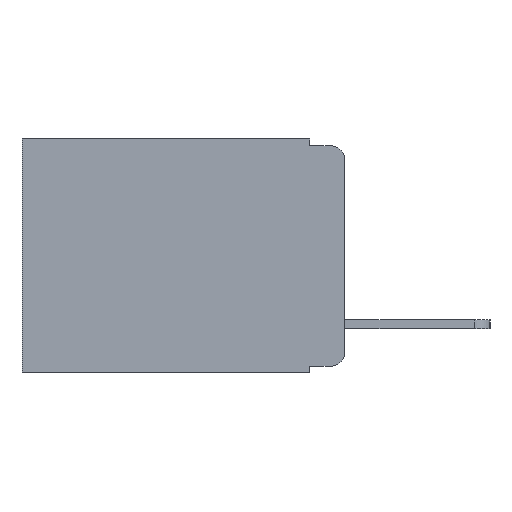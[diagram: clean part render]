
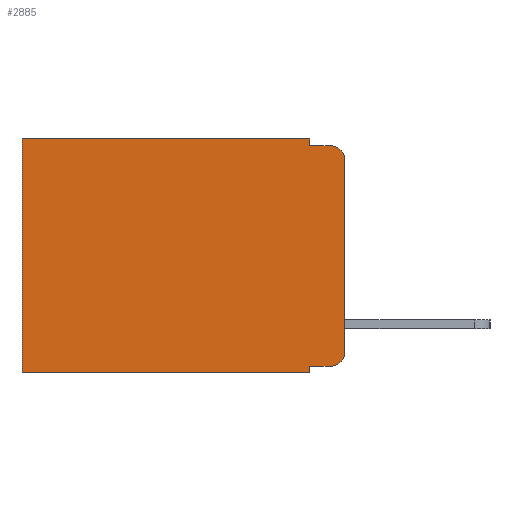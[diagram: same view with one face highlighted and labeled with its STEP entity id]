
A CAD part, left-side view. The second image highlights one B-rep face of the part: STEP entity #2885.
In plain terms, the highlighted planar face has unit normal (-1, 0, 0).
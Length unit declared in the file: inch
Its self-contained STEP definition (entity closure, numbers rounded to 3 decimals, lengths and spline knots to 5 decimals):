
#58 = ORIENTED_EDGE ( 'NONE', *, *, #12656, .T. ) ;
#78 = VECTOR ( 'NONE', #8382, 39.37008 ) ;
#124 = EDGE_CURVE ( 'NONE', #10309, #8480, #2674, .T. ) ;
#230 = CARTESIAN_POINT ( 'NONE',  ( 0.298, 0., 0. ) ) ;
#416 = CARTESIAN_POINT ( 'NONE',  ( 0.298, 0., -0.343 ) ) ;
#528 = DIRECTION ( 'NONE',  ( 0., 1., 0. ) ) ;
#673 = VERTEX_POINT ( 'NONE', #12947 ) ;
#687 = CARTESIAN_POINT ( 'NONE',  ( 0.298, 0., -0.03 ) ) ;
#918 = CARTESIAN_POINT ( 'NONE',  ( 0.298, 0.051, 0. ) ) ;
#926 = CARTESIAN_POINT ( 'NONE',  ( 0.298, 0.051, 0. ) ) ;
#1571 = CARTESIAN_POINT ( 'NONE',  ( 0.298, 0.473, 0. ) ) ;
#2151 = LINE ( 'NONE', #5682, #7761 ) ;
#2384 = CARTESIAN_POINT ( 'NONE',  ( 0.298, 0.02, -0.03 ) ) ;
#2459 = DIRECTION ( 'NONE',  ( -1., 0., 0. ) ) ;
#2674 = LINE ( 'NONE', #3791, #10426 ) ;
#2885 = ADVANCED_FACE ( 'NONE', ( #9297 ), #5388, .F. ) ;
#3448 = DIRECTION ( 'NONE',  ( 0., 0., -1. ) ) ;
#3570 = ORIENTED_EDGE ( 'NONE', *, *, #11837, .T. ) ;
#3630 = DIRECTION ( 'NONE',  ( 0., -1., 0. ) ) ;
#3791 = CARTESIAN_POINT ( 'NONE',  ( 0.298, 0., 0. ) ) ;
#4272 = CIRCLE ( 'NONE', #10037, 0.02 ) ;
#4332 = CARTESIAN_POINT ( 'NONE',  ( 0.298, 0.051, 0. ) ) ;
#4416 = EDGE_LOOP ( 'NONE', ( #10687, #7862, #9593, #11970, #8514, #12189, #11569, #4531, #58, #3570 ) ) ;
#4449 = VERTEX_POINT ( 'NONE', #12935 ) ;
#4519 = VECTOR ( 'NONE', #4658, 39.37008 ) ;
#4531 = ORIENTED_EDGE ( 'NONE', *, *, #6214, .F. ) ;
#4658 = DIRECTION ( 'NONE',  ( 0., 0., -1. ) ) ;
#4736 = VERTEX_POINT ( 'NONE', #6519 ) ;
#5169 = CARTESIAN_POINT ( 'NONE',  ( 0.298, 0.051, -0.01 ) ) ;
#5209 = LINE ( 'NONE', #230, #10890 ) ;
#5315 = VERTEX_POINT ( 'NONE', #10993 ) ;
#5388 = PLANE ( 'NONE',  #5704 ) ;
#5412 = EDGE_CURVE ( 'NONE', #10309, #5315, #9362, .T. ) ;
#5477 = VERTEX_POINT ( 'NONE', #9401 ) ;
#5626 = EDGE_CURVE ( 'NONE', #673, #10710, #12557, .T. ) ;
#5682 = CARTESIAN_POINT ( 'NONE',  ( 0.298, 0.051, -0.333 ) ) ;
#5704 = AXIS2_PLACEMENT_3D ( 'NONE', #12985, #11744, #10931 ) ;
#5815 = CARTESIAN_POINT ( 'NONE',  ( 0.298, 0.473, 0. ) ) ;
#6214 = EDGE_CURVE ( 'NONE', #4736, #673, #8204, .T. ) ;
#6451 = DIRECTION ( 'NONE',  ( 0., 0., -1. ) ) ;
#6519 = CARTESIAN_POINT ( 'NONE',  ( 0.298, 0.051, -0.333 ) ) ;
#6553 = VECTOR ( 'NONE', #12726, 39.37008 ) ;
#7052 = VECTOR ( 'NONE', #9134, 39.37008 ) ;
#7289 = EDGE_CURVE ( 'NONE', #8480, #10710, #10128, .T. ) ;
#7761 = VECTOR ( 'NONE', #3630, 39.37008 ) ;
#7862 = ORIENTED_EDGE ( 'NONE', *, *, #13173, .T. ) ;
#8204 = LINE ( 'NONE', #918, #10313 ) ;
#8382 = DIRECTION ( 'NONE',  ( 0., -1., 0. ) ) ;
#8480 = VERTEX_POINT ( 'NONE', #5815 ) ;
#8514 = ORIENTED_EDGE ( 'NONE', *, *, #124, .T. ) ;
#8770 = CARTESIAN_POINT ( 'NONE',  ( 0.298, 0.02, -0.313 ) ) ;
#9134 = DIRECTION ( 'NONE',  ( 0., 1., 0. ) ) ;
#9161 = VERTEX_POINT ( 'NONE', #12059 ) ;
#9297 = FACE_OUTER_BOUND ( 'NONE', #4416, .T. ) ;
#9362 = LINE ( 'NONE', #4332, #6553 ) ;
#9401 = CARTESIAN_POINT ( 'NONE',  ( 0.298, 0.02, -0.01 ) ) ;
#9593 = ORIENTED_EDGE ( 'NONE', *, *, #13001, .F. ) ;
#9752 = DIRECTION ( 'NONE',  ( -1., 0., 0. ) ) ;
#9827 = DIRECTION ( 'NONE',  ( 0., 0., -1. ) ) ;
#9939 = AXIS2_PLACEMENT_3D ( 'NONE', #8770, #2459, #9827 ) ;
#10037 = AXIS2_PLACEMENT_3D ( 'NONE', #2384, #9752, #3448 ) ;
#10128 = LINE ( 'NONE', #1571, #4519 ) ;
#10309 = VERTEX_POINT ( 'NONE', #926 ) ;
#10313 = VECTOR ( 'NONE', #12939, 39.37008 ) ;
#10426 = VECTOR ( 'NONE', #528, 39.37008 ) ;
#10687 = ORIENTED_EDGE ( 'NONE', *, *, #12455, .F. ) ;
#10710 = VERTEX_POINT ( 'NONE', #10971 ) ;
#10890 = VECTOR ( 'NONE', #6451, 39.37008 ) ;
#10931 = DIRECTION ( 'NONE',  ( 0., 0., -1. ) ) ;
#10971 = CARTESIAN_POINT ( 'NONE',  ( 0.298, 0.473, -0.343 ) ) ;
#10993 = CARTESIAN_POINT ( 'NONE',  ( 0.298, 0.051, -0.01 ) ) ;
#11478 = LINE ( 'NONE', #5169, #78 ) ;
#11569 = ORIENTED_EDGE ( 'NONE', *, *, #5626, .F. ) ;
#11744 = DIRECTION ( 'NONE',  ( 1., 0., 0. ) ) ;
#11837 = EDGE_CURVE ( 'NONE', #4449, #9161, #13195, .T. ) ;
#11970 = ORIENTED_EDGE ( 'NONE', *, *, #5412, .F. ) ;
#12059 = CARTESIAN_POINT ( 'NONE',  ( 0.298, 0., -0.313 ) ) ;
#12189 = ORIENTED_EDGE ( 'NONE', *, *, #7289, .T. ) ;
#12455 = EDGE_CURVE ( 'NONE', #12779, #9161, #5209, .T. ) ;
#12557 = LINE ( 'NONE', #416, #7052 ) ;
#12656 = EDGE_CURVE ( 'NONE', #4736, #4449, #2151, .T. ) ;
#12726 = DIRECTION ( 'NONE',  ( 0., 0., -1. ) ) ;
#12779 = VERTEX_POINT ( 'NONE', #687 ) ;
#12935 = CARTESIAN_POINT ( 'NONE',  ( 0.298, 0.02, -0.333 ) ) ;
#12939 = DIRECTION ( 'NONE',  ( 0., 0., -1. ) ) ;
#12947 = CARTESIAN_POINT ( 'NONE',  ( 0.298, 0.051, -0.343 ) ) ;
#12985 = CARTESIAN_POINT ( 'NONE',  ( 0.298, 0., 0. ) ) ;
#13001 = EDGE_CURVE ( 'NONE', #5315, #5477, #11478, .T. ) ;
#13173 = EDGE_CURVE ( 'NONE', #12779, #5477, #4272, .T. ) ;
#13195 = CIRCLE ( 'NONE', #9939, 0.02 ) ;
